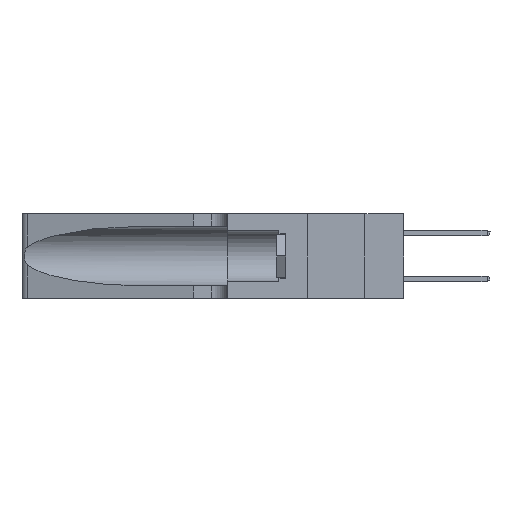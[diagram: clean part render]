
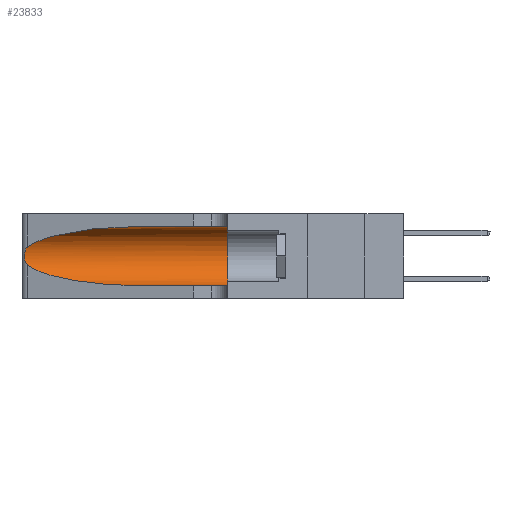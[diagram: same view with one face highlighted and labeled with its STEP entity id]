
A CAD part, left-side view. The second image highlights one B-rep face of the part: STEP entity #23833.
In plain terms, the highlighted cylindrical face has radius 3.308 mm (diameter 6.617 mm), a partial arc.
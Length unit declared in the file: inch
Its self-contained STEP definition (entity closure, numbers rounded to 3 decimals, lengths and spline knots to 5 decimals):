
#639 = CARTESIAN_POINT ( 'NONE',  ( 0.1305, 0.35, 0.185 ) ) ;
#709 = ORIENTED_EDGE ( 'NONE', *, *, #22280, .F. ) ;
#748 = CARTESIAN_POINT ( 'NONE',  ( 0.26075, 1.23896, 0.19203 ) ) ;
#1071 = CARTESIAN_POINT ( 'NONE',  ( 0.25555, 1.22993, 0.14849 ) ) ;
#1237 = CARTESIAN_POINT ( 'NONE',  ( 0.25487, 1.22718, 0.22369 ) ) ;
#1522 = DIRECTION ( 'NONE',  ( 0., 0., -1. ) ) ;
#1622 = VERTEX_POINT ( 'NONE', #5526 ) ;
#1969 = EDGE_CURVE ( 'NONE', #28276, #43806, #5308, .T. ) ;
#2533 = CARTESIAN_POINT ( 'NONE',  ( 0.1305, 0.35, 0.31525 ) ) ;
#3146 = CARTESIAN_POINT ( 'NONE',  ( 0.25487, 1.22718, 0.14631 ) ) ;
#4789 = DIRECTION ( 'NONE',  ( 0., -1., 0. ) ) ;
#4973 = CARTESIAN_POINT ( 'NONE',  ( 0.25487, 1.22718, 0.14631 ) ) ;
#5308 = B_SPLINE_CURVE_WITH_KNOTS ( 'NONE', 3,
 ( #1237, #14415, #24603, #35266, #38556, #34952, #748, #38248, #35425, #18030, #10926, #42321, #1071, #25068 ),
 .UNSPECIFIED., .F., .F.,
 ( 4, 2, 2, 2, 2, 2, 4 ),
 ( 0., 0.00027, 0.00053, 0.00107, 0.0016, 0.00187, 0.00214 ),
 .UNSPECIFIED. ) ;
#5526 = CARTESIAN_POINT ( 'NONE',  ( 0.1305, 0.72297, 0.05475 ) ) ;
#6993 = CARTESIAN_POINT ( 'NONE',  ( 0.18966, 0.96281, 0.05475 ) ) ;
#7553 = FACE_OUTER_BOUND ( 'NONE', #16469, .T. ) ;
#8090 = CARTESIAN_POINT ( 'NONE',  ( 0.25487, 1.22718, 0.22369 ) ) ;
#8796 = CARTESIAN_POINT ( 'NONE',  ( 0.1305, 1.61858, 0.05475 ) ) ;
#10593 = EDGE_CURVE ( 'NONE', #30846, #28276, #22629, .T. ) ;
#10828 = VERTEX_POINT ( 'NONE', #2533 ) ;
#10857 = LINE ( 'NONE', #8796, #39393 ) ;
#10926 = CARTESIAN_POINT ( 'NONE',  ( 0.25789, 1.23486, 0.15765 ) ) ;
#10986 = DIRECTION ( 'NONE',  ( 0., 0., 1. ) ) ;
#11089 = CARTESIAN_POINT ( 'NONE',  ( 0.1305, 1.61858, 0.31525 ) ) ;
#11145 = CARTESIAN_POINT ( 'NONE',  ( 0.1305, 0.72297, 0.31525 ) ) ;
#14314 = DIRECTION ( 'NONE',  ( 0., 1., 0. ) ) ;
#14415 = CARTESIAN_POINT ( 'NONE',  ( 0.25555, 1.22994, 0.2215 ) ) ;
#14937 = CARTESIAN_POINT ( 'NONE',  ( 0.25487, 1.22718, 0.22369 ) ) ;
#16469 = EDGE_LOOP ( 'NONE', ( #38146, #33979, #33042, #36544, #19168, #709 ) ) ;
#17212 = CARTESIAN_POINT ( 'NONE',  ( 0.1305, 0.72297, 0.31525 ) ) ;
#18030 = CARTESIAN_POINT ( 'NONE',  ( 0.25856, 1.23593, 0.16098 ) ) ;
#18186 = DIRECTION ( 'NONE',  ( 0., -1., 0. ) ) ;
#19168 = ORIENTED_EDGE ( 'NONE', *, *, #40835, .F. ) ;
#20114 = AXIS2_PLACEMENT_3D ( 'NONE', #39178, #25044, #1522 ) ;
#21181 = CIRCLE ( 'NONE', #33026, 0.13025 ) ;
#22280 = EDGE_CURVE ( 'NONE', #30846, #10828, #43198, .T. ) ;
#22629 =( BOUNDED_CURVE ( )  B_SPLINE_CURVE ( 3, ( #17212, #31711, #27668, #14937 ),
 .UNSPECIFIED., .F., .F. ) 
 B_SPLINE_CURVE_WITH_KNOTS ( ( 4, 4 ),
 ( 1.5708, 2.84003 ),
 .UNSPECIFIED. ) 
 CURVE ( )  GEOMETRIC_REPRESENTATION_ITEM ( )  RATIONAL_B_SPLINE_CURVE ( ( 1., 0.87, 0.87, 1. ) ) 
 REPRESENTATION_ITEM ( '' )  );
#23165 = CYLINDRICAL_SURFACE ( 'NONE', #20114, 0.13025 ) ;
#23833 = ADVANCED_FACE ( 'NONE', ( #7553 ), #23165, .F. ) ;
#24603 = CARTESIAN_POINT ( 'NONE',  ( 0.25639, 1.23184, 0.21858 ) ) ;
#25044 = DIRECTION ( 'NONE',  ( 0., -1., 0. ) ) ;
#25068 = CARTESIAN_POINT ( 'NONE',  ( 0.25487, 1.22718, 0.14631 ) ) ;
#26917 = EDGE_CURVE ( 'NONE', #1622, #37321, #10857, .T. ) ;
#27114 = CARTESIAN_POINT ( 'NONE',  ( 0.2373, 1.15595, 0.08982 ) ) ;
#27668 = CARTESIAN_POINT ( 'NONE',  ( 0.2373, 1.15595, 0.28018 ) ) ;
#28276 = VERTEX_POINT ( 'NONE', #8090 ) ;
#28712 = EDGE_CURVE ( 'NONE', #43806, #1622, #30563, .T. ) ;
#28744 = CARTESIAN_POINT ( 'NONE',  ( 0.1305, 0.35, 0.05475 ) ) ;
#30563 =( BOUNDED_CURVE ( )  B_SPLINE_CURVE ( 3, ( #3146, #27114, #6993, #34035 ),
 .UNSPECIFIED., .F., .F. ) 
 B_SPLINE_CURVE_WITH_KNOTS ( ( 4, 4 ),
 ( 3.44316, 4.71239 ),
 .UNSPECIFIED. ) 
 CURVE ( )  GEOMETRIC_REPRESENTATION_ITEM ( )  RATIONAL_B_SPLINE_CURVE ( ( 1., 0.87, 0.87, 1. ) ) 
 REPRESENTATION_ITEM ( '' )  );
#30846 = VERTEX_POINT ( 'NONE', #11145 ) ;
#31711 = CARTESIAN_POINT ( 'NONE',  ( 0.18966, 0.96281, 0.31525 ) ) ;
#33026 = AXIS2_PLACEMENT_3D ( 'NONE', #639, #14314, #10986 ) ;
#33042 = ORIENTED_EDGE ( 'NONE', *, *, #28712, .T. ) ;
#33979 = ORIENTED_EDGE ( 'NONE', *, *, #1969, .T. ) ;
#34035 = CARTESIAN_POINT ( 'NONE',  ( 0.1305, 0.72297, 0.05475 ) ) ;
#34952 = CARTESIAN_POINT ( 'NONE',  ( 0.26018, 1.23835, 0.19895 ) ) ;
#35266 = CARTESIAN_POINT ( 'NONE',  ( 0.25787, 1.23484, 0.2124 ) ) ;
#35425 = CARTESIAN_POINT ( 'NONE',  ( 0.26017, 1.23833, 0.17102 ) ) ;
#36544 = ORIENTED_EDGE ( 'NONE', *, *, #26917, .T. ) ;
#37321 = VERTEX_POINT ( 'NONE', #28744 ) ;
#38146 = ORIENTED_EDGE ( 'NONE', *, *, #10593, .T. ) ;
#38248 = CARTESIAN_POINT ( 'NONE',  ( 0.26075, 1.23896, 0.178 ) ) ;
#38556 = CARTESIAN_POINT ( 'NONE',  ( 0.25854, 1.2359, 0.20912 ) ) ;
#39178 = CARTESIAN_POINT ( 'NONE',  ( 0.1305, 1.61858, 0.185 ) ) ;
#39393 = VECTOR ( 'NONE', #4789, 39.37008 ) ;
#40835 = EDGE_CURVE ( 'NONE', #10828, #37321, #21181, .T. ) ;
#41051 = VECTOR ( 'NONE', #18186, 39.37008 ) ;
#42321 = CARTESIAN_POINT ( 'NONE',  ( 0.25639, 1.23186, 0.15144 ) ) ;
#43198 = LINE ( 'NONE', #11089, #41051 ) ;
#43806 = VERTEX_POINT ( 'NONE', #4973 ) ;
